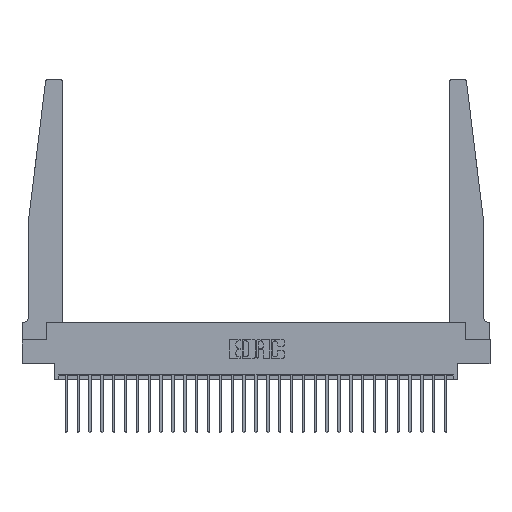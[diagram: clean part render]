
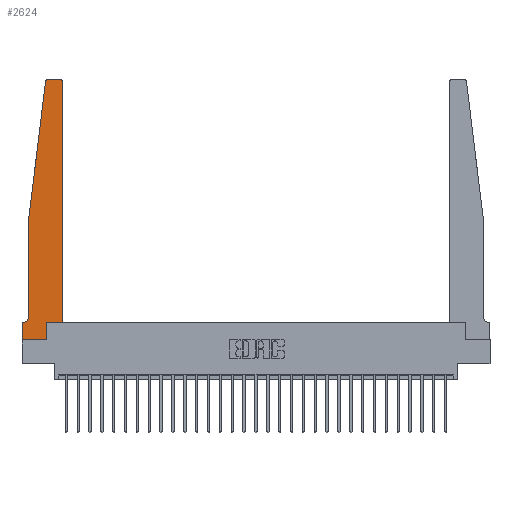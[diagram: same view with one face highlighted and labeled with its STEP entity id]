
A CAD part, top view. The second image highlights one B-rep face of the part: STEP entity #2624.
In plain terms, the highlighted planar face has unit normal (0, 0, 1).
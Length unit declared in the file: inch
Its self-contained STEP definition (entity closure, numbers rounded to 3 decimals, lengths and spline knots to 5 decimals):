
#255 = EDGE_CURVE ( 'NONE', #21593, #9469, #18028, .T. ) ;
#689 = CARTESIAN_POINT ( 'NONE',  ( 0.065, 0.2375, 0.37 ) ) ;
#905 = VECTOR ( 'NONE', #11463, 39.37008 ) ;
#1440 = CARTESIAN_POINT ( 'NONE',  ( 0.015, 0.1875, 0.37 ) ) ;
#1520 = DIRECTION ( 'NONE',  ( 0., 1., 0. ) ) ;
#1630 = ORIENTED_EDGE ( 'NONE', *, *, #7569, .T. ) ;
#2486 = CARTESIAN_POINT ( 'NONE',  ( 0.065, 1.25, 0.37 ) ) ;
#2624 = ADVANCED_FACE ( 'NONE', ( #4885 ), #22401, .T. ) ;
#2890 = VERTEX_POINT ( 'NONE', #13135 ) ;
#3180 = ORIENTED_EDGE ( 'NONE', *, *, #255, .T. ) ;
#3337 = CARTESIAN_POINT ( 'NONE',  ( 0.2605, 0.18, 0.37 ) ) ;
#3391 = ORIENTED_EDGE ( 'NONE', *, *, #21431, .T. ) ;
#4753 = EDGE_CURVE ( 'NONE', #13759, #12936, #13821, .T. ) ;
#4850 = DIRECTION ( 'NONE',  ( 1., 0., 0. ) ) ;
#4885 = FACE_OUTER_BOUND ( 'NONE', #13047, .T. ) ;
#4961 = CARTESIAN_POINT ( 'NONE',  ( 0.065, 1.25, 0.37 ) ) ;
#4980 = CARTESIAN_POINT ( 'NONE',  ( 0.395, 2.72, 0.37 ) ) ;
#4984 = ORIENTED_EDGE ( 'NONE', *, *, #25681, .T. ) ;
#5091 = DIRECTION ( 'NONE',  ( 0., 0., 1. ) ) ;
#5842 = EDGE_CURVE ( 'NONE', #20895, #2890, #17792, .T. ) ;
#6151 = ORIENTED_EDGE ( 'NONE', *, *, #16792, .T. ) ;
#6987 = CARTESIAN_POINT ( 'NONE',  ( 0., 0., 0.37 ) ) ;
#7093 = VECTOR ( 'NONE', #9147, 39.37008 ) ;
#7143 = AXIS2_PLACEMENT_3D ( 'NONE', #17455, #24476, #12340 ) ;
#7144 = DIRECTION ( 'NONE',  ( 1., 0., 0. ) ) ;
#7493 = CARTESIAN_POINT ( 'NONE',  ( 0.425, 0.18, 0.37 ) ) ;
#7569 = EDGE_CURVE ( 'NONE', #17554, #14793, #20382, .T. ) ;
#7983 = CARTESIAN_POINT ( 'NONE',  ( 0.2605, 0., 0.37 ) ) ;
#8833 = VECTOR ( 'NONE', #26979, 39.37008 ) ;
#8994 = CARTESIAN_POINT ( 'NONE',  ( 0.425, 0.18, 0.37 ) ) ;
#9147 = DIRECTION ( 'NONE',  ( 1., 0., 0. ) ) ;
#9172 = ORIENTED_EDGE ( 'NONE', *, *, #20170, .T. ) ;
#9469 = VERTEX_POINT ( 'NONE', #1440 ) ;
#9797 = ORIENTED_EDGE ( 'NONE', *, *, #4753, .T. ) ;
#10007 = EDGE_CURVE ( 'NONE', #15893, #10475, #19014, .T. ) ;
#10140 = LINE ( 'NONE', #16921, #20144 ) ;
#10475 = VERTEX_POINT ( 'NONE', #25480 ) ;
#11463 = DIRECTION ( 'NONE',  ( -1., 0., 0. ) ) ;
#11633 = VERTEX_POINT ( 'NONE', #25407 ) ;
#11662 = ORIENTED_EDGE ( 'NONE', *, *, #14627, .T. ) ;
#12340 = DIRECTION ( 'NONE',  ( -1., 0., 0. ) ) ;
#12655 = DIRECTION ( 'NONE',  ( 0., -1., 0. ) ) ;
#12936 = VERTEX_POINT ( 'NONE', #3337 ) ;
#12983 = VECTOR ( 'NONE', #13429, 39.37008 ) ;
#13047 = EDGE_LOOP ( 'NONE', ( #9172, #15271, #4984, #15077, #3180, #25817, #15259, #11662, #9797, #3391, #1630, #6151 ) ) ;
#13135 = CARTESIAN_POINT ( 'NONE',  ( 0.24675, 2.72367, 0.37 ) ) ;
#13161 = CIRCLE ( 'NONE', #19243, 0.03 ) ;
#13347 = VECTOR ( 'NONE', #22075, 39.37008 ) ;
#13429 = DIRECTION ( 'NONE',  ( -1., 0., 0. ) ) ;
#13759 = VERTEX_POINT ( 'NONE', #7983 ) ;
#13821 = LINE ( 'NONE', #14196, #8833 ) ;
#13899 = DIRECTION ( 'NONE',  ( 1., 0., 0. ) ) ;
#14196 = CARTESIAN_POINT ( 'NONE',  ( 0.2605, 0.18, 0.37 ) ) ;
#14583 = VERTEX_POINT ( 'NONE', #2486 ) ;
#14627 = EDGE_CURVE ( 'NONE', #10475, #13759, #25449, .T. ) ;
#14687 = LINE ( 'NONE', #4961, #13347 ) ;
#14710 = VECTOR ( 'NONE', #1520, 39.37008 ) ;
#14793 = VERTEX_POINT ( 'NONE', #22582 ) ;
#15077 = ORIENTED_EDGE ( 'NONE', *, *, #17185, .T. ) ;
#15259 = ORIENTED_EDGE ( 'NONE', *, *, #10007, .T. ) ;
#15271 = ORIENTED_EDGE ( 'NONE', *, *, #5842, .T. ) ;
#15564 = CARTESIAN_POINT ( 'NONE',  ( 0.065, 0.1875, 0.37 ) ) ;
#15893 = VERTEX_POINT ( 'NONE', #19213 ) ;
#16261 = LINE ( 'NONE', #8994, #16916 ) ;
#16792 = EDGE_CURVE ( 'NONE', #14793, #11633, #13161, .T. ) ;
#16916 = VECTOR ( 'NONE', #4850, 39.37008 ) ;
#16921 = CARTESIAN_POINT ( 'NONE',  ( 0.065, 1.25, 0.37 ) ) ;
#17185 = EDGE_CURVE ( 'NONE', #14583, #21593, #10140, .T. ) ;
#17455 = CARTESIAN_POINT ( 'NONE',  ( 0.015, 0.2375, 0.37 ) ) ;
#17554 = VERTEX_POINT ( 'NONE', #7493 ) ;
#17789 = CARTESIAN_POINT ( 'NONE',  ( 0.25, 2.75, 0.37 ) ) ;
#17792 = CIRCLE ( 'NONE', #26329, 0.03 ) ;
#17858 = CARTESIAN_POINT ( 'NONE',  ( 0.27653, 2.72, 0.37 ) ) ;
#17965 = LINE ( 'NONE', #17789, #905 ) ;
#18028 = CIRCLE ( 'NONE', #7143, 0.05 ) ;
#18032 = DIRECTION ( 'NONE',  ( 0., -1., 0. ) ) ;
#18344 = VECTOR ( 'NONE', #18032, 39.37008 ) ;
#18631 = LINE ( 'NONE', #15564, #12983 ) ;
#19014 = LINE ( 'NONE', #24377, #18344 ) ;
#19213 = CARTESIAN_POINT ( 'NONE',  ( 0., 0.1875, 0.37 ) ) ;
#19243 = AXIS2_PLACEMENT_3D ( 'NONE', #4980, #19916, #7144 ) ;
#19916 = DIRECTION ( 'NONE',  ( 0., 0., 1. ) ) ;
#20012 = DIRECTION ( 'NONE',  ( 1., 0., 0. ) ) ;
#20102 = CARTESIAN_POINT ( 'NONE',  ( 0.27653, 2.75, 0.37 ) ) ;
#20132 = EDGE_CURVE ( 'NONE', #9469, #15893, #18631, .T. ) ;
#20144 = VECTOR ( 'NONE', #12655, 39.37008 ) ;
#20170 = EDGE_CURVE ( 'NONE', #11633, #20895, #17965, .T. ) ;
#20382 = LINE ( 'NONE', #22840, #14710 ) ;
#20895 = VERTEX_POINT ( 'NONE', #20102 ) ;
#21431 = EDGE_CURVE ( 'NONE', #12936, #17554, #16261, .T. ) ;
#21593 = VERTEX_POINT ( 'NONE', #689 ) ;
#22075 = DIRECTION ( 'NONE',  ( -0.122, -0.992, 0. ) ) ;
#22401 = PLANE ( 'NONE',  #25395 ) ;
#22582 = CARTESIAN_POINT ( 'NONE',  ( 0.425, 2.72, 0.37 ) ) ;
#22840 = CARTESIAN_POINT ( 'NONE',  ( 0.425, 0.18, 0.37 ) ) ;
#24377 = CARTESIAN_POINT ( 'NONE',  ( 0., 0., 0.37 ) ) ;
#24476 = DIRECTION ( 'NONE',  ( 0., 0., -1. ) ) ;
#24514 = CARTESIAN_POINT ( 'NONE',  ( 0., 0.1875, 0.37 ) ) ;
#25395 = AXIS2_PLACEMENT_3D ( 'NONE', #24514, #26668, #13899 ) ;
#25407 = CARTESIAN_POINT ( 'NONE',  ( 0.395, 2.75, 0.37 ) ) ;
#25449 = LINE ( 'NONE', #6987, #7093 ) ;
#25480 = CARTESIAN_POINT ( 'NONE',  ( 0., 0., 0.37 ) ) ;
#25681 = EDGE_CURVE ( 'NONE', #2890, #14583, #14687, .T. ) ;
#25817 = ORIENTED_EDGE ( 'NONE', *, *, #20132, .T. ) ;
#26329 = AXIS2_PLACEMENT_3D ( 'NONE', #17858, #5091, #20012 ) ;
#26668 = DIRECTION ( 'NONE',  ( 0., 0., 1. ) ) ;
#26979 = DIRECTION ( 'NONE',  ( 0., 1., 0. ) ) ;
